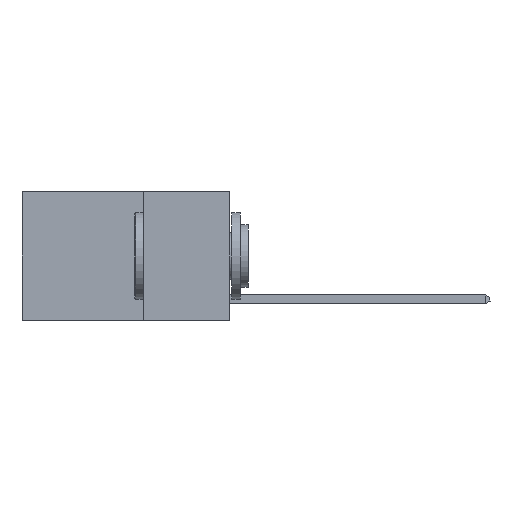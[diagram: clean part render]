
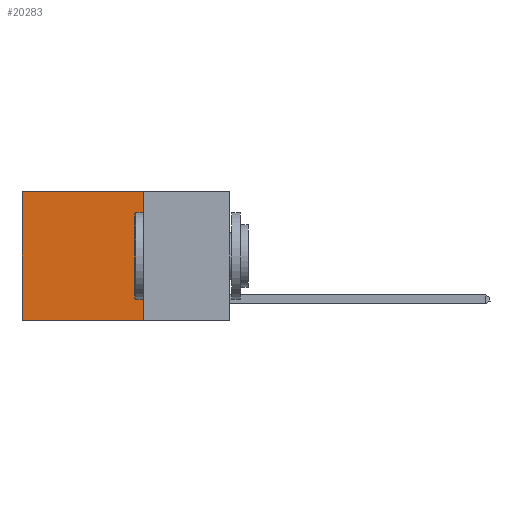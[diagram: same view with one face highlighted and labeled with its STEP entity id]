
A CAD part, left-side view. The second image highlights one B-rep face of the part: STEP entity #20283.
In plain terms, the highlighted planar face has unit normal (-1, 0, 0).
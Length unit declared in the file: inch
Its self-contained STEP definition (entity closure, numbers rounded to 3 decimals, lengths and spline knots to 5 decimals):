
#153 = PLANE ( 'NONE',  #21848 ) ;
#623 = VERTEX_POINT ( 'NONE', #18181 ) ;
#1272 = VECTOR ( 'NONE', #20964, 39.37008 ) ;
#1667 = EDGE_CURVE ( 'NONE', #19691, #623, #16970, .T. ) ;
#2789 = ORIENTED_EDGE ( 'NONE', *, *, #1667, .F. ) ;
#3548 = CARTESIAN_POINT ( 'NONE',  ( 0.2625, 0.25, -0.37 ) ) ;
#4014 = DIRECTION ( 'NONE',  ( 0., 1., 0. ) ) ;
#4918 = VECTOR ( 'NONE', #18189, 39.37008 ) ;
#5479 = EDGE_CURVE ( 'NONE', #11827, #19691, #13140, .T. ) ;
#5734 = VERTEX_POINT ( 'NONE', #11470 ) ;
#6194 = CARTESIAN_POINT ( 'NONE',  ( 0.2625, 0.25, 0. ) ) ;
#7306 = EDGE_CURVE ( 'NONE', #5734, #623, #8975, .T. ) ;
#8975 = LINE ( 'NONE', #9734, #4918 ) ;
#9734 = CARTESIAN_POINT ( 'NONE',  ( 0.2625, 0.6, 0. ) ) ;
#10315 = DIRECTION ( 'NONE',  ( 0., 0., -1. ) ) ;
#10851 = CARTESIAN_POINT ( 'NONE',  ( 0.2625, 0.25, -0.37 ) ) ;
#11470 = CARTESIAN_POINT ( 'NONE',  ( 0.2625, 0.6, 0. ) ) ;
#11636 = EDGE_CURVE ( 'NONE', #11827, #5734, #22330, .T. ) ;
#11812 = ORIENTED_EDGE ( 'NONE', *, *, #5479, .F. ) ;
#11827 = VERTEX_POINT ( 'NONE', #6194 ) ;
#12185 = DIRECTION ( 'NONE',  ( 1., 0., 0. ) ) ;
#12274 = VECTOR ( 'NONE', #4014, 39.37008 ) ;
#12548 = CARTESIAN_POINT ( 'NONE',  ( 0.2625, 0.25, 0. ) ) ;
#13140 = LINE ( 'NONE', #18723, #1272 ) ;
#13247 = EDGE_LOOP ( 'NONE', ( #13708, #2789, #11812, #16143 ) ) ;
#13708 = ORIENTED_EDGE ( 'NONE', *, *, #7306, .T. ) ;
#16143 = ORIENTED_EDGE ( 'NONE', *, *, #11636, .T. ) ;
#16970 = LINE ( 'NONE', #10851, #19128 ) ;
#18181 = CARTESIAN_POINT ( 'NONE',  ( 0.2625, 0.6, -0.37 ) ) ;
#18189 = DIRECTION ( 'NONE',  ( 0., 0., -1. ) ) ;
#18723 = CARTESIAN_POINT ( 'NONE',  ( 0.2625, 0.25, 0. ) ) ;
#18861 = FACE_OUTER_BOUND ( 'NONE', #13247, .T. ) ;
#19128 = VECTOR ( 'NONE', #19386, 39.37008 ) ;
#19386 = DIRECTION ( 'NONE',  ( 0., 1., 0. ) ) ;
#19691 = VERTEX_POINT ( 'NONE', #3548 ) ;
#20283 = ADVANCED_FACE ( 'NONE', ( #18861 ), #153, .F. ) ;
#20678 = CARTESIAN_POINT ( 'NONE',  ( 0.2625, 0.25, 0. ) ) ;
#20964 = DIRECTION ( 'NONE',  ( 0., 0., -1. ) ) ;
#21848 = AXIS2_PLACEMENT_3D ( 'NONE', #20678, #12185, #10315 ) ;
#22330 = LINE ( 'NONE', #12548, #12274 ) ;
